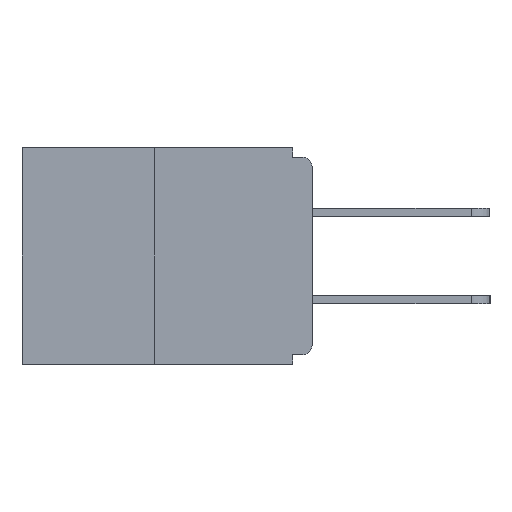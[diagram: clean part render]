
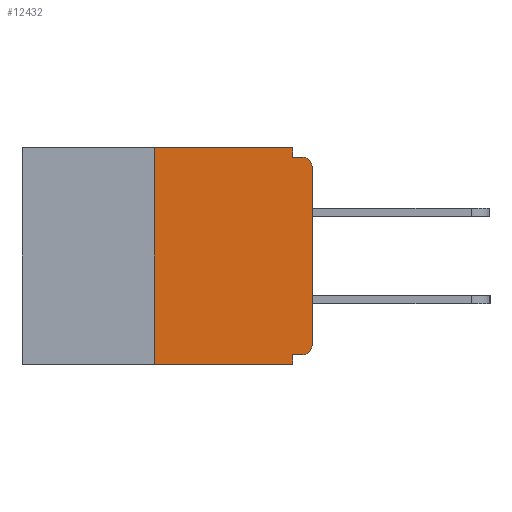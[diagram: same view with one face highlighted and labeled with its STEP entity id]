
A CAD part, left-side view. The second image highlights one B-rep face of the part: STEP entity #12432.
In plain terms, the highlighted planar face has unit normal (-1, 0, 0).
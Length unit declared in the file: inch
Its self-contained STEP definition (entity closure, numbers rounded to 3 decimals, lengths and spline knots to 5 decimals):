
#40 = DIRECTION ( 'NONE',  ( -1., 0., 0. ) ) ;
#141 = LINE ( 'NONE', #9985, #12352 ) ;
#482 = CARTESIAN_POINT ( 'NONE',  ( 0., 0.46, 0. ) ) ;
#695 = LINE ( 'NONE', #10073, #3366 ) ;
#832 = EDGE_CURVE ( 'NONE', #9579, #12255, #695, .T. ) ;
#870 = DIRECTION ( 'NONE',  ( -1., 0., 0. ) ) ;
#965 = ORIENTED_EDGE ( 'NONE', *, *, #5032, .F. ) ;
#1008 = LINE ( 'NONE', #12308, #6403 ) ;
#1086 = CARTESIAN_POINT ( 'NONE',  ( 0., 0., -0.313 ) ) ;
#1389 = AXIS2_PLACEMENT_3D ( 'NONE', #15627, #870, #14060 ) ;
#1463 = LINE ( 'NONE', #6237, #15915 ) ;
#1575 = EDGE_LOOP ( 'NONE', ( #3031, #4050, #15648, #2107, #4755, #13601, #2161, #2391, #7587, #965 ) ) ;
#1697 = VECTOR ( 'NONE', #14167, 39.37008 ) ;
#1860 = DIRECTION ( 'NONE',  ( 0., -1., 0. ) ) ;
#2107 = ORIENTED_EDGE ( 'NONE', *, *, #3118, .F. ) ;
#2161 = ORIENTED_EDGE ( 'NONE', *, *, #6239, .T. ) ;
#2391 = ORIENTED_EDGE ( 'NONE', *, *, #6633, .T. ) ;
#2610 = CIRCLE ( 'NONE', #13750, 0.015 ) ;
#3031 = ORIENTED_EDGE ( 'NONE', *, *, #10920, .F. ) ;
#3085 = VERTEX_POINT ( 'NONE', #9662 ) ;
#3118 = EDGE_CURVE ( 'NONE', #3489, #3774, #1008, .T. ) ;
#3266 = VERTEX_POINT ( 'NONE', #1086 ) ;
#3366 = VECTOR ( 'NONE', #10030, 39.37008 ) ;
#3489 = VERTEX_POINT ( 'NONE', #6462 ) ;
#3698 = DIRECTION ( 'NONE',  ( 0., 0., -1. ) ) ;
#3774 = VERTEX_POINT ( 'NONE', #12267 ) ;
#3833 = DIRECTION ( 'NONE',  ( 0., 1., 0. ) ) ;
#4050 = ORIENTED_EDGE ( 'NONE', *, *, #4956, .F. ) ;
#4158 = PLANE ( 'NONE',  #13222 ) ;
#4190 = LINE ( 'NONE', #11682, #1697 ) ;
#4481 = CARTESIAN_POINT ( 'NONE',  ( 0., 0.46, -0.343 ) ) ;
#4586 = VECTOR ( 'NONE', #9652, 39.37008 ) ;
#4755 = ORIENTED_EDGE ( 'NONE', *, *, #7962, .F. ) ;
#4956 = EDGE_CURVE ( 'NONE', #15839, #5306, #8833, .T. ) ;
#5032 = EDGE_CURVE ( 'NONE', #14969, #9579, #4190, .T. ) ;
#5269 = CARTESIAN_POINT ( 'NONE',  ( 0., 0.031, 0. ) ) ;
#5306 = VERTEX_POINT ( 'NONE', #14531 ) ;
#5345 = DIRECTION ( 'NONE',  ( 0., 0., -1. ) ) ;
#5402 = DIRECTION ( 'NONE',  ( 1., 0., 0. ) ) ;
#6235 = CARTESIAN_POINT ( 'NONE',  ( 0., 0.031, -0.015 ) ) ;
#6237 = CARTESIAN_POINT ( 'NONE',  ( 0., 0.46, 0. ) ) ;
#6239 = EDGE_CURVE ( 'NONE', #3266, #7819, #15775, .T. ) ;
#6403 = VECTOR ( 'NONE', #13605, 39.37008 ) ;
#6462 = CARTESIAN_POINT ( 'NONE',  ( 0., 0.031, -0.328 ) ) ;
#6633 = EDGE_CURVE ( 'NONE', #7819, #12255, #14028, .T. ) ;
#6865 = VECTOR ( 'NONE', #1860, 39.37008 ) ;
#7420 = EDGE_CURVE ( 'NONE', #15839, #3774, #8775, .T. ) ;
#7525 = CARTESIAN_POINT ( 'NONE',  ( 0., 0.015, -0.313 ) ) ;
#7587 = ORIENTED_EDGE ( 'NONE', *, *, #832, .F. ) ;
#7819 = VERTEX_POINT ( 'NONE', #11432 ) ;
#7962 = EDGE_CURVE ( 'NONE', #3085, #3489, #141, .T. ) ;
#8041 = VECTOR ( 'NONE', #15398, 39.37008 ) ;
#8775 = LINE ( 'NONE', #4481, #6865 ) ;
#8833 = LINE ( 'NONE', #12754, #8041 ) ;
#9020 = CARTESIAN_POINT ( 'NONE',  ( 0., 0.015, -0.015 ) ) ;
#9579 = VERTEX_POINT ( 'NONE', #6235 ) ;
#9652 = DIRECTION ( 'NONE',  ( 0., 0., 1. ) ) ;
#9662 = CARTESIAN_POINT ( 'NONE',  ( 0., 0.015, -0.328 ) ) ;
#9696 = CARTESIAN_POINT ( 'NONE',  ( 0., 0., 0. ) ) ;
#9985 = CARTESIAN_POINT ( 'NONE',  ( 0., 0., -0.328 ) ) ;
#10030 = DIRECTION ( 'NONE',  ( 0., -1., 0. ) ) ;
#10073 = CARTESIAN_POINT ( 'NONE',  ( 0., 0., -0.015 ) ) ;
#10920 = EDGE_CURVE ( 'NONE', #5306, #14969, #1463, .T. ) ;
#11432 = CARTESIAN_POINT ( 'NONE',  ( 0., 0., -0.03 ) ) ;
#11682 = CARTESIAN_POINT ( 'NONE',  ( 0., 0.031, 0. ) ) ;
#12255 = VERTEX_POINT ( 'NONE', #9020 ) ;
#12267 = CARTESIAN_POINT ( 'NONE',  ( 0., 0.031, -0.343 ) ) ;
#12308 = CARTESIAN_POINT ( 'NONE',  ( 0., 0.031, -0.343 ) ) ;
#12352 = VECTOR ( 'NONE', #3833, 39.37008 ) ;
#12432 = ADVANCED_FACE ( 'NONE', ( #15728 ), #4158, .F. ) ;
#12754 = CARTESIAN_POINT ( 'NONE',  ( 0., 0.25, 0. ) ) ;
#13222 = AXIS2_PLACEMENT_3D ( 'NONE', #482, #5402, #5345 ) ;
#13555 = EDGE_CURVE ( 'NONE', #3085, #3266, #2610, .T. ) ;
#13601 = ORIENTED_EDGE ( 'NONE', *, *, #13555, .T. ) ;
#13605 = DIRECTION ( 'NONE',  ( 0., 0., -1. ) ) ;
#13750 = AXIS2_PLACEMENT_3D ( 'NONE', #7525, #40, #3698 ) ;
#14028 = CIRCLE ( 'NONE', #1389, 0.015 ) ;
#14060 = DIRECTION ( 'NONE',  ( 0., 0., -1. ) ) ;
#14167 = DIRECTION ( 'NONE',  ( 0., 0., -1. ) ) ;
#14318 = CARTESIAN_POINT ( 'NONE',  ( 0., 0.25, -0.343 ) ) ;
#14531 = CARTESIAN_POINT ( 'NONE',  ( 0., 0.25, 0. ) ) ;
#14864 = DIRECTION ( 'NONE',  ( 0., -1., 0. ) ) ;
#14969 = VERTEX_POINT ( 'NONE', #5269 ) ;
#15398 = DIRECTION ( 'NONE',  ( 0., 0., 1. ) ) ;
#15627 = CARTESIAN_POINT ( 'NONE',  ( 0., 0.015, -0.03 ) ) ;
#15648 = ORIENTED_EDGE ( 'NONE', *, *, #7420, .T. ) ;
#15728 = FACE_OUTER_BOUND ( 'NONE', #1575, .T. ) ;
#15775 = LINE ( 'NONE', #9696, #4586 ) ;
#15839 = VERTEX_POINT ( 'NONE', #14318 ) ;
#15915 = VECTOR ( 'NONE', #14864, 39.37008 ) ;
